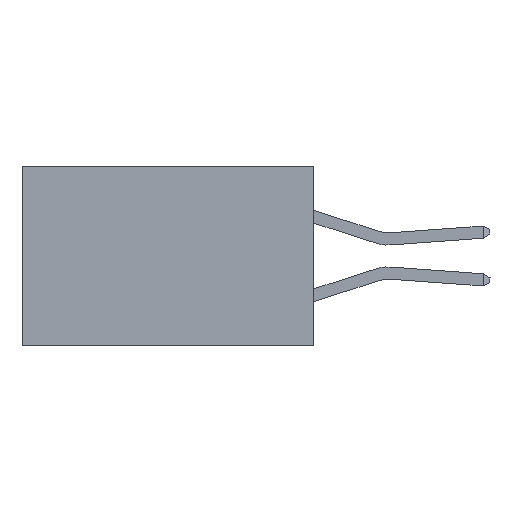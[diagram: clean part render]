
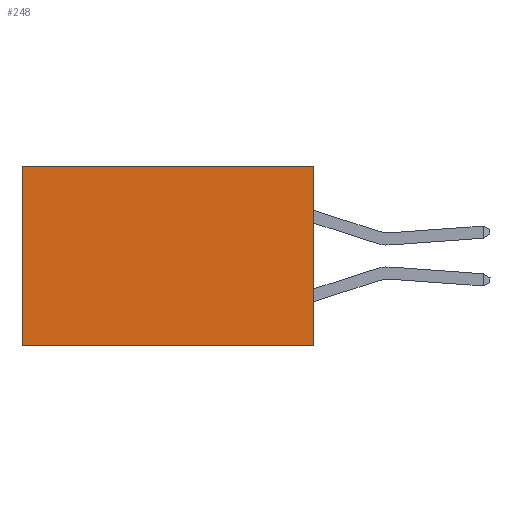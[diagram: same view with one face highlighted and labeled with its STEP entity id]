
A CAD part, left-side view. The second image highlights one B-rep face of the part: STEP entity #248.
In plain terms, the highlighted planar face has unit normal (-1, 0, 0).
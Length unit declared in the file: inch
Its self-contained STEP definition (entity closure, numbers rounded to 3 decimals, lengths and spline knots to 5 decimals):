
#69 = VERTEX_POINT ( 'NONE', #15500 ) ;
#248 = ADVANCED_FACE ( 'NONE', ( #17682 ), #16260, .F. ) ;
#1434 = DIRECTION ( 'NONE',  ( 0., 0., -1. ) ) ;
#2169 = CARTESIAN_POINT ( 'NONE',  ( 0.2875, 0., -0.37 ) ) ;
#2353 = ORIENTED_EDGE ( 'NONE', *, *, #27506, .F. ) ;
#2963 = DIRECTION ( 'NONE',  ( 0., 0., -1. ) ) ;
#3323 = CARTESIAN_POINT ( 'NONE',  ( 0.2875, 0.6, 0. ) ) ;
#3375 = DIRECTION ( 'NONE',  ( 0., 0., -1. ) ) ;
#3508 = ORIENTED_EDGE ( 'NONE', *, *, #23424, .T. ) ;
#3654 = EDGE_LOOP ( 'NONE', ( #3508, #2353, #16198, #20987 ) ) ;
#4829 = LINE ( 'NONE', #14483, #26804 ) ;
#5044 = VERTEX_POINT ( 'NONE', #22615 ) ;
#8069 = CARTESIAN_POINT ( 'NONE',  ( 0.2875, 0., 0. ) ) ;
#9007 = EDGE_CURVE ( 'NONE', #69, #18232, #28228, .T. ) ;
#10087 = VECTOR ( 'NONE', #10458, 39.37008 ) ;
#10458 = DIRECTION ( 'NONE',  ( 0., 1., 0. ) ) ;
#12250 = LINE ( 'NONE', #2169, #27216 ) ;
#13682 = LINE ( 'NONE', #8069, #27259 ) ;
#14483 = CARTESIAN_POINT ( 'NONE',  ( 0.2875, 0.6, 0. ) ) ;
#15500 = CARTESIAN_POINT ( 'NONE',  ( 0.2875, 0., 0. ) ) ;
#16198 = ORIENTED_EDGE ( 'NONE', *, *, #20518, .F. ) ;
#16224 = DIRECTION ( 'NONE',  ( 0., 1., 0. ) ) ;
#16260 = PLANE ( 'NONE',  #21314 ) ;
#17682 = FACE_OUTER_BOUND ( 'NONE', #3654, .T. ) ;
#18127 = CARTESIAN_POINT ( 'NONE',  ( 0.2875, 0., -0.37 ) ) ;
#18232 = VERTEX_POINT ( 'NONE', #3323 ) ;
#18733 = DIRECTION ( 'NONE',  ( 1., 0., 0. ) ) ;
#19255 = VERTEX_POINT ( 'NONE', #18127 ) ;
#20518 = EDGE_CURVE ( 'NONE', #69, #19255, #13682, .T. ) ;
#20987 = ORIENTED_EDGE ( 'NONE', *, *, #9007, .T. ) ;
#21314 = AXIS2_PLACEMENT_3D ( 'NONE', #27276, #18733, #2963 ) ;
#21399 = CARTESIAN_POINT ( 'NONE',  ( 0.2875, 0., 0. ) ) ;
#22615 = CARTESIAN_POINT ( 'NONE',  ( 0.2875, 0.6, -0.37 ) ) ;
#23424 = EDGE_CURVE ( 'NONE', #18232, #5044, #4829, .T. ) ;
#26804 = VECTOR ( 'NONE', #3375, 39.37008 ) ;
#27216 = VECTOR ( 'NONE', #16224, 39.37008 ) ;
#27259 = VECTOR ( 'NONE', #1434, 39.37008 ) ;
#27276 = CARTESIAN_POINT ( 'NONE',  ( 0.2875, 0., 0. ) ) ;
#27506 = EDGE_CURVE ( 'NONE', #19255, #5044, #12250, .T. ) ;
#28228 = LINE ( 'NONE', #21399, #10087 ) ;
